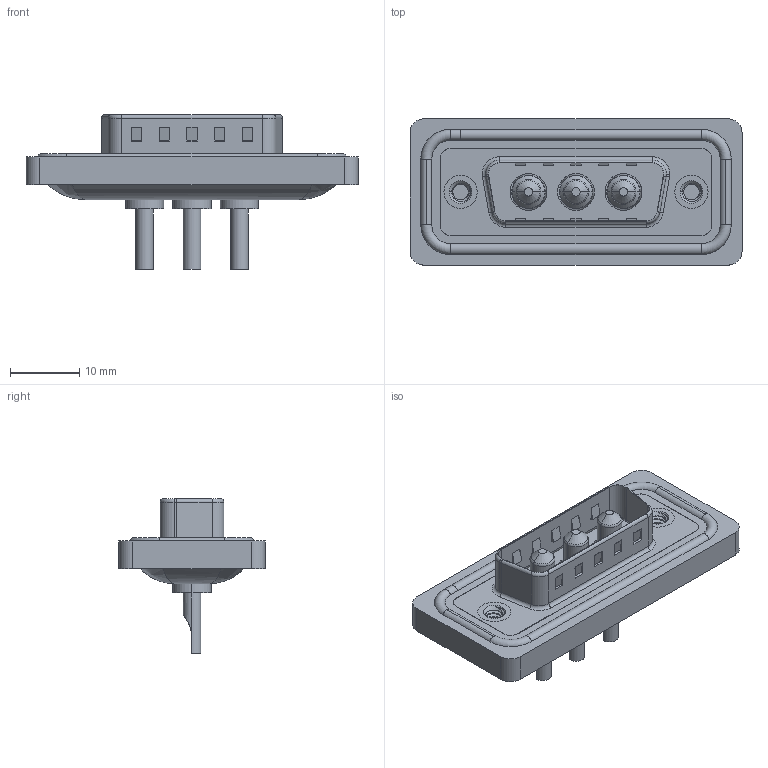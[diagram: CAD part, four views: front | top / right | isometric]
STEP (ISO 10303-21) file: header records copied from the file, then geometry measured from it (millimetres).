
FILE_DESCRIPTION (( 'STEP AP203' ), '1' );
FILE_NAME ('627W3W3-122-1N2.STEP', '2024-03-20T14:12:00', ( '' ), ( '' ), 'SwSTEP 2.0', 'SolidWorks 2023', '' );
FILE_SCHEMA (( 'CONFIG_CONTROL_DESIGN' ));
Length unit declared in the file: millimetre
Products named in the file (7): 627Combo Shell Rear_15 Contacts; Power Pin_10A SC; 627Combo Shell Front_15 Contacts; 627W3W3-122-1N2; 627Combo Waterproof Housing_15 Contacts; 627Combo Threaded Rivet_2; 627Combo Housing_3W3
Assembly tree (9 placements, depth 2):
  627W3W3-122-1N2
    627Combo Housing_3W3
    627Combo Waterproof Housing_15 Contacts
    627Combo Shell Rear_15 Contacts
    627Combo Shell Front_15 Contacts
    627Combo Threaded Rivet_2  x2
    Power Pin_10A SC  x3
Bounding box: 47.9 x 21.1 x 22.3 mm (x, y, z)
Volume: 5577.4 mm3; surface area: 8896.6 mm2
Topology: 13 solids, 13 shells, 579 faces, 1417 edges, 880 vertices
Faces by surface type: cylinder 250, plane 213, torus 70, cone 33, bspline 13
Entity records: 16560 total; most frequent: CARTESIAN_POINT 4350, DIRECTION 2488, ORIENTED_EDGE 2320, EDGE_CURVE 1160, AXIS2_PLACEMENT_3D 929, VERTEX_POINT 730, VECTOR 630, LINE 630
